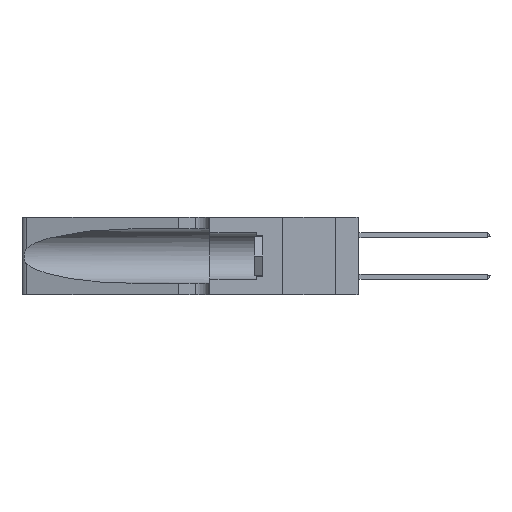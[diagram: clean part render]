
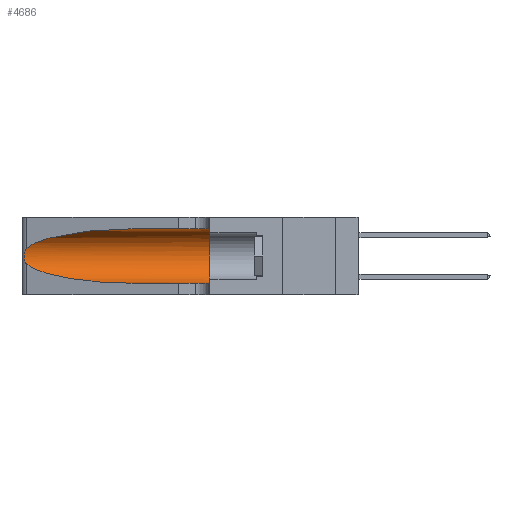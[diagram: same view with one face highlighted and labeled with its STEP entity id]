
A CAD part, left-side view. The second image highlights one B-rep face of the part: STEP entity #4686.
In plain terms, the highlighted cylindrical face has radius 3.308 mm (diameter 6.617 mm), a partial arc.
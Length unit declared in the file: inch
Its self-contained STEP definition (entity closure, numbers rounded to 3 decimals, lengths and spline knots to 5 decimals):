
#334 = LINE ( 'NONE', #24712, #15605 ) ;
#670 = AXIS2_PLACEMENT_3D ( 'NONE', #9267, #22379, #22143 ) ;
#1084 = DIRECTION ( 'NONE',  ( 0., 0., 1. ) ) ;
#2651 = FACE_OUTER_BOUND ( 'NONE', #5786, .T. ) ;
#2799 = AXIS2_PLACEMENT_3D ( 'NONE', #31923, #16448, #1084 ) ;
#2945 = CARTESIAN_POINT ( 'NONE',  ( 0.2373, 1.15595, 0.08982 ) ) ;
#3117 = CARTESIAN_POINT ( 'NONE',  ( 0.25639, 1.23186, 0.15144 ) ) ;
#3437 = CARTESIAN_POINT ( 'NONE',  ( 0.25487, 1.22718, 0.22369 ) ) ;
#4155 = CARTESIAN_POINT ( 'NONE',  ( 0.1305, 0.72297, 0.05475 ) ) ;
#4686 = ADVANCED_FACE ( 'NONE', ( #2651 ), #32028, .F. ) ;
#5786 = EDGE_LOOP ( 'NONE', ( #8632, #18993, #16127, #26693, #20446, #20710 ) ) ;
#6002 = CARTESIAN_POINT ( 'NONE',  ( 0.25639, 1.23184, 0.21858 ) ) ;
#6124 = CARTESIAN_POINT ( 'NONE',  ( 0.26075, 1.23896, 0.19203 ) ) ;
#7072 = CARTESIAN_POINT ( 'NONE',  ( 0.2373, 1.15595, 0.28018 ) ) ;
#7315 = CARTESIAN_POINT ( 'NONE',  ( 0.1305, 0.72297, 0.31525 ) ) ;
#8632 = ORIENTED_EDGE ( 'NONE', *, *, #9251, .T. ) ;
#8983 = VERTEX_POINT ( 'NONE', #13933 ) ;
#9251 = EDGE_CURVE ( 'NONE', #8983, #12388, #18177, .T. ) ;
#9267 = CARTESIAN_POINT ( 'NONE',  ( 0.1305, 1.61858, 0.185 ) ) ;
#9460 = VERTEX_POINT ( 'NONE', #4155 ) ;
#9538 = CARTESIAN_POINT ( 'NONE',  ( 0.18966, 0.96281, 0.31525 ) ) ;
#10238 =( BOUNDED_CURVE ( )  B_SPLINE_CURVE ( 3, ( #12876, #2945, #10710, #20959 ),
 .UNSPECIFIED., .F., .F. ) 
 B_SPLINE_CURVE_WITH_KNOTS ( ( 4, 4 ),
 ( 3.44316, 4.71239 ),
 .UNSPECIFIED. ) 
 CURVE ( )  GEOMETRIC_REPRESENTATION_ITEM ( )  RATIONAL_B_SPLINE_CURVE ( ( 1., 0.87, 0.87, 1. ) ) 
 REPRESENTATION_ITEM ( '' )  );
#10710 = CARTESIAN_POINT ( 'NONE',  ( 0.18966, 0.96281, 0.05475 ) ) ;
#10770 = CARTESIAN_POINT ( 'NONE',  ( 0.26075, 1.23896, 0.178 ) ) ;
#11610 = EDGE_CURVE ( 'NONE', #15731, #30091, #19826, .T. ) ;
#11971 = DIRECTION ( 'NONE',  ( 0., -1., 0. ) ) ;
#12388 = VERTEX_POINT ( 'NONE', #31408 ) ;
#12876 = CARTESIAN_POINT ( 'NONE',  ( 0.25487, 1.22718, 0.14631 ) ) ;
#13338 = CARTESIAN_POINT ( 'NONE',  ( 0.26017, 1.23833, 0.17102 ) ) ;
#13557 = CARTESIAN_POINT ( 'NONE',  ( 0.1305, 1.61858, 0.05475 ) ) ;
#13909 = CARTESIAN_POINT ( 'NONE',  ( 0.1305, 0.35, 0.31525 ) ) ;
#13933 = CARTESIAN_POINT ( 'NONE',  ( 0.1305, 0.72297, 0.31525 ) ) ;
#14551 = CARTESIAN_POINT ( 'NONE',  ( 0.25487, 1.22718, 0.22369 ) ) ;
#14726 = B_SPLINE_CURVE_WITH_KNOTS ( 'NONE', 3,
 ( #3437, #16315, #6002, #21029, #21479, #18452, #6124, #10770, #13338, #31345, #15889, #3117, #26216, #21593 ),
 .UNSPECIFIED., .F., .F.,
 ( 4, 2, 2, 2, 2, 2, 4 ),
 ( 0., 0.00027, 0.00053, 0.00107, 0.0016, 0.00187, 0.00214 ),
 .UNSPECIFIED. ) ;
#15148 = EDGE_CURVE ( 'NONE', #12388, #15840, #14726, .T. ) ;
#15605 = VECTOR ( 'NONE', #11971, 39.37008 ) ;
#15731 = VERTEX_POINT ( 'NONE', #13909 ) ;
#15840 = VERTEX_POINT ( 'NONE', #21512 ) ;
#15889 = CARTESIAN_POINT ( 'NONE',  ( 0.25789, 1.23486, 0.15765 ) ) ;
#16127 = ORIENTED_EDGE ( 'NONE', *, *, #27140, .T. ) ;
#16315 = CARTESIAN_POINT ( 'NONE',  ( 0.25555, 1.22994, 0.2215 ) ) ;
#16448 = DIRECTION ( 'NONE',  ( 0., 1., 0. ) ) ;
#18177 =( BOUNDED_CURVE ( )  B_SPLINE_CURVE ( 3, ( #7315, #9538, #7072, #14551 ),
 .UNSPECIFIED., .F., .F. ) 
 B_SPLINE_CURVE_WITH_KNOTS ( ( 4, 4 ),
 ( 1.5708, 2.84003 ),
 .UNSPECIFIED. ) 
 CURVE ( )  GEOMETRIC_REPRESENTATION_ITEM ( )  RATIONAL_B_SPLINE_CURVE ( ( 1., 0.87, 0.87, 1. ) ) 
 REPRESENTATION_ITEM ( '' )  );
#18452 = CARTESIAN_POINT ( 'NONE',  ( 0.26018, 1.23835, 0.19895 ) ) ;
#18993 = ORIENTED_EDGE ( 'NONE', *, *, #15148, .T. ) ;
#19826 = CIRCLE ( 'NONE', #2799, 0.13025 ) ;
#20113 = EDGE_CURVE ( 'NONE', #9460, #30091, #32570, .T. ) ;
#20446 = ORIENTED_EDGE ( 'NONE', *, *, #11610, .F. ) ;
#20710 = ORIENTED_EDGE ( 'NONE', *, *, #23297, .F. ) ;
#20959 = CARTESIAN_POINT ( 'NONE',  ( 0.1305, 0.72297, 0.05475 ) ) ;
#21029 = CARTESIAN_POINT ( 'NONE',  ( 0.25787, 1.23484, 0.2124 ) ) ;
#21479 = CARTESIAN_POINT ( 'NONE',  ( 0.25854, 1.2359, 0.20912 ) ) ;
#21512 = CARTESIAN_POINT ( 'NONE',  ( 0.25487, 1.22718, 0.14631 ) ) ;
#21593 = CARTESIAN_POINT ( 'NONE',  ( 0.25487, 1.22718, 0.14631 ) ) ;
#22143 = DIRECTION ( 'NONE',  ( 0., 0., -1. ) ) ;
#22379 = DIRECTION ( 'NONE',  ( 0., -1., 0. ) ) ;
#23297 = EDGE_CURVE ( 'NONE', #8983, #15731, #334, .T. ) ;
#24712 = CARTESIAN_POINT ( 'NONE',  ( 0.1305, 1.61858, 0.31525 ) ) ;
#25659 = VECTOR ( 'NONE', #29120, 39.37008 ) ;
#26216 = CARTESIAN_POINT ( 'NONE',  ( 0.25555, 1.22993, 0.14849 ) ) ;
#26693 = ORIENTED_EDGE ( 'NONE', *, *, #20113, .T. ) ;
#27140 = EDGE_CURVE ( 'NONE', #15840, #9460, #10238, .T. ) ;
#28955 = CARTESIAN_POINT ( 'NONE',  ( 0.1305, 0.35, 0.05475 ) ) ;
#29120 = DIRECTION ( 'NONE',  ( 0., -1., 0. ) ) ;
#30091 = VERTEX_POINT ( 'NONE', #28955 ) ;
#31345 = CARTESIAN_POINT ( 'NONE',  ( 0.25856, 1.23593, 0.16098 ) ) ;
#31408 = CARTESIAN_POINT ( 'NONE',  ( 0.25487, 1.22718, 0.22369 ) ) ;
#31923 = CARTESIAN_POINT ( 'NONE',  ( 0.1305, 0.35, 0.185 ) ) ;
#32028 = CYLINDRICAL_SURFACE ( 'NONE', #670, 0.13025 ) ;
#32570 = LINE ( 'NONE', #13557, #25659 ) ;
